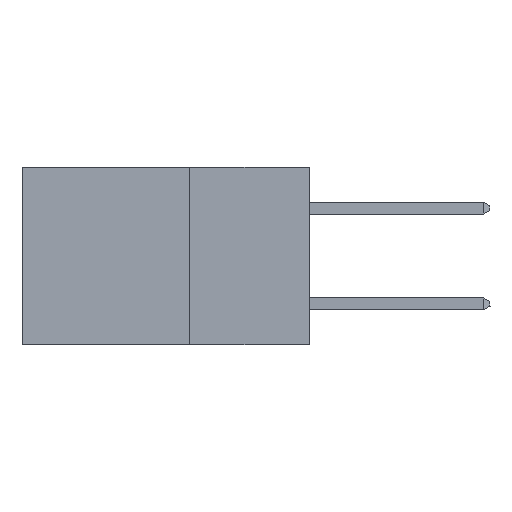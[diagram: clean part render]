
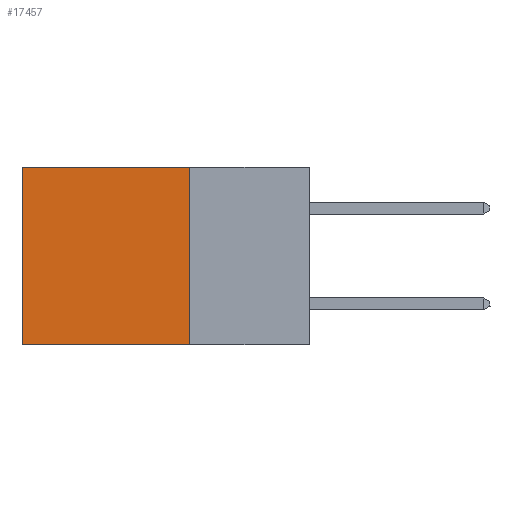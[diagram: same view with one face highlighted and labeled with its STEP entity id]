
A CAD part, left-side view. The second image highlights one B-rep face of the part: STEP entity #17457.
In plain terms, the highlighted planar face has unit normal (-1, 0, 0).
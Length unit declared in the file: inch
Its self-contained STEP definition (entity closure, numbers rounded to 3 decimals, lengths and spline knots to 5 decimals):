
#1170 = PLANE ( 'NONE',  #5015 ) ;
#1912 = DIRECTION ( 'NONE',  ( 1., 0., 0. ) ) ;
#4266 = CARTESIAN_POINT ( 'NONE',  ( 0.2875, 0.6, 0. ) ) ;
#4636 = VERTEX_POINT ( 'NONE', #22176 ) ;
#4757 = VERTEX_POINT ( 'NONE', #5997 ) ;
#4935 = EDGE_CURVE ( 'NONE', #16484, #4636, #5317, .T. ) ;
#5015 = AXIS2_PLACEMENT_3D ( 'NONE', #19780, #1912, #19874 ) ;
#5245 = ORIENTED_EDGE ( 'NONE', *, *, #7479, .F. ) ;
#5317 = LINE ( 'NONE', #4266, #10596 ) ;
#5814 = LINE ( 'NONE', #10842, #16757 ) ;
#5997 = CARTESIAN_POINT ( 'NONE',  ( 0.2875, 0.25, 0. ) ) ;
#6243 = DIRECTION ( 'NONE',  ( 0., 0., -1. ) ) ;
#6766 = DIRECTION ( 'NONE',  ( 0., 1., 0. ) ) ;
#7479 = EDGE_CURVE ( 'NONE', #21985, #4636, #5814, .T. ) ;
#7571 = FACE_OUTER_BOUND ( 'NONE', #21215, .T. ) ;
#7847 = VECTOR ( 'NONE', #9542, 39.37008 ) ;
#8530 = ORIENTED_EDGE ( 'NONE', *, *, #10247, .F. ) ;
#9390 = CARTESIAN_POINT ( 'NONE',  ( 0.2875, 0.25, -0.37 ) ) ;
#9542 = DIRECTION ( 'NONE',  ( 0., 0., -1. ) ) ;
#9596 = VECTOR ( 'NONE', #6766, 39.37008 ) ;
#10167 = CARTESIAN_POINT ( 'NONE',  ( 0.2875, 0.6, 0. ) ) ;
#10247 = EDGE_CURVE ( 'NONE', #4757, #21985, #13113, .T. ) ;
#10456 = ORIENTED_EDGE ( 'NONE', *, *, #4935, .T. ) ;
#10596 = VECTOR ( 'NONE', #6243, 39.37008 ) ;
#10842 = CARTESIAN_POINT ( 'NONE',  ( 0.2875, 0.25, -0.37 ) ) ;
#13078 = DIRECTION ( 'NONE',  ( 0., 1., 0. ) ) ;
#13113 = LINE ( 'NONE', #13691, #7847 ) ;
#13691 = CARTESIAN_POINT ( 'NONE',  ( 0.2875, 0.25, 0. ) ) ;
#14294 = LINE ( 'NONE', #18668, #9596 ) ;
#16484 = VERTEX_POINT ( 'NONE', #10167 ) ;
#16757 = VECTOR ( 'NONE', #13078, 39.37008 ) ;
#17457 = ADVANCED_FACE ( 'NONE', ( #7571 ), #1170, .F. ) ;
#18537 = ORIENTED_EDGE ( 'NONE', *, *, #20835, .T. ) ;
#18668 = CARTESIAN_POINT ( 'NONE',  ( 0.2875, 0.25, 0. ) ) ;
#19780 = CARTESIAN_POINT ( 'NONE',  ( 0.2875, 0.25, 0. ) ) ;
#19874 = DIRECTION ( 'NONE',  ( 0., 0., -1. ) ) ;
#20835 = EDGE_CURVE ( 'NONE', #4757, #16484, #14294, .T. ) ;
#21215 = EDGE_LOOP ( 'NONE', ( #10456, #5245, #8530, #18537 ) ) ;
#21985 = VERTEX_POINT ( 'NONE', #9390 ) ;
#22176 = CARTESIAN_POINT ( 'NONE',  ( 0.2875, 0.6, -0.37 ) ) ;
